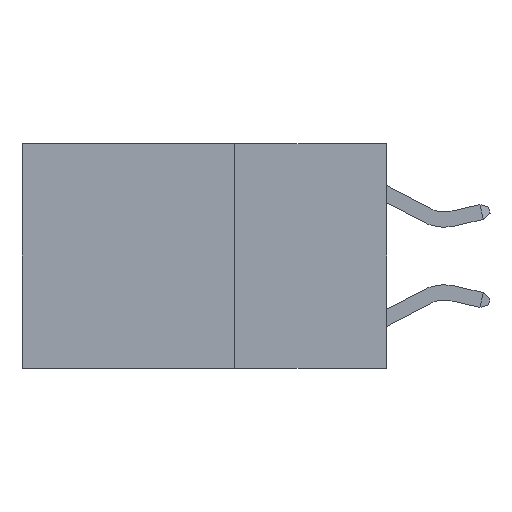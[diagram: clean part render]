
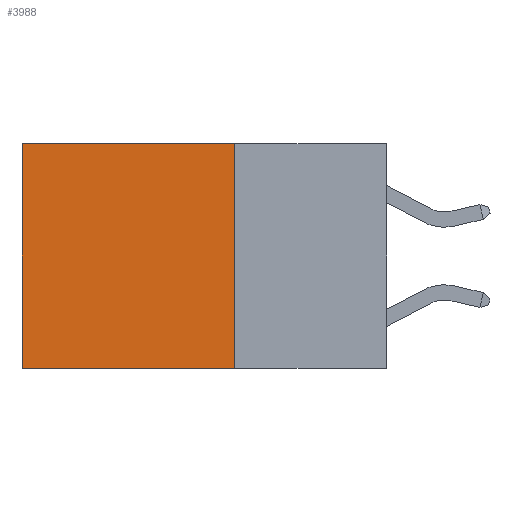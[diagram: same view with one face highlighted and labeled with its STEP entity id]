
A CAD part, left-side view. The second image highlights one B-rep face of the part: STEP entity #3988.
In plain terms, the highlighted planar face has unit normal (-1, 0, 0).
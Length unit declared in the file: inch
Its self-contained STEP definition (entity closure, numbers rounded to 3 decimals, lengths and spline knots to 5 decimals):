
#758 = CARTESIAN_POINT ( 'NONE',  ( 0.2625, 0.25, -0.37 ) ) ;
#828 = DIRECTION ( 'NONE',  ( 0., 1., 0. ) ) ;
#864 = CARTESIAN_POINT ( 'NONE',  ( 0.2625, 0.25, -0.37 ) ) ;
#1581 = VERTEX_POINT ( 'NONE', #10968 ) ;
#1677 = LINE ( 'NONE', #864, #5433 ) ;
#1871 = LINE ( 'NONE', #6033, #2143 ) ;
#2143 = VECTOR ( 'NONE', #828, 39.37008 ) ;
#2173 = VECTOR ( 'NONE', #6238, 39.37008 ) ;
#2270 = EDGE_CURVE ( 'NONE', #2665, #1581, #1871, .T. ) ;
#2665 = VERTEX_POINT ( 'NONE', #10612 ) ;
#2736 = ORIENTED_EDGE ( 'NONE', *, *, #2270, .T. ) ;
#3120 = LINE ( 'NONE', #11526, #2173 ) ;
#3223 = ORIENTED_EDGE ( 'NONE', *, *, #11574, .F. ) ;
#3988 = ADVANCED_FACE ( 'NONE', ( #10984 ), #13194, .F. ) ;
#4980 = DIRECTION ( 'NONE',  ( 0., 0., -1. ) ) ;
#5433 = VECTOR ( 'NONE', #5841, 39.37008 ) ;
#5841 = DIRECTION ( 'NONE',  ( 0., 1., 0. ) ) ;
#6033 = CARTESIAN_POINT ( 'NONE',  ( 0.2625, 0.25, 0. ) ) ;
#6082 = CARTESIAN_POINT ( 'NONE',  ( 0.2625, 0.6, 0. ) ) ;
#6238 = DIRECTION ( 'NONE',  ( 0., 0., -1. ) ) ;
#7022 = ORIENTED_EDGE ( 'NONE', *, *, #11970, .F. ) ;
#7939 = VERTEX_POINT ( 'NONE', #758 ) ;
#7969 = CARTESIAN_POINT ( 'NONE',  ( 0.2625, 0.25, 0. ) ) ;
#8218 = LINE ( 'NONE', #6082, #13345 ) ;
#8654 = VERTEX_POINT ( 'NONE', #12236 ) ;
#9948 = DIRECTION ( 'NONE',  ( 1., 0., 0. ) ) ;
#10101 = DIRECTION ( 'NONE',  ( 0., 0., -1. ) ) ;
#10612 = CARTESIAN_POINT ( 'NONE',  ( 0.2625, 0.25, 0. ) ) ;
#10968 = CARTESIAN_POINT ( 'NONE',  ( 0.2625, 0.6, 0. ) ) ;
#10984 = FACE_OUTER_BOUND ( 'NONE', #12523, .T. ) ;
#11460 = AXIS2_PLACEMENT_3D ( 'NONE', #7969, #9948, #10101 ) ;
#11526 = CARTESIAN_POINT ( 'NONE',  ( 0.2625, 0.25, 0. ) ) ;
#11574 = EDGE_CURVE ( 'NONE', #7939, #8654, #1677, .T. ) ;
#11970 = EDGE_CURVE ( 'NONE', #2665, #7939, #3120, .T. ) ;
#11995 = ORIENTED_EDGE ( 'NONE', *, *, #12132, .T. ) ;
#12132 = EDGE_CURVE ( 'NONE', #1581, #8654, #8218, .T. ) ;
#12236 = CARTESIAN_POINT ( 'NONE',  ( 0.2625, 0.6, -0.37 ) ) ;
#12523 = EDGE_LOOP ( 'NONE', ( #11995, #3223, #7022, #2736 ) ) ;
#13194 = PLANE ( 'NONE',  #11460 ) ;
#13345 = VECTOR ( 'NONE', #4980, 39.37008 ) ;
